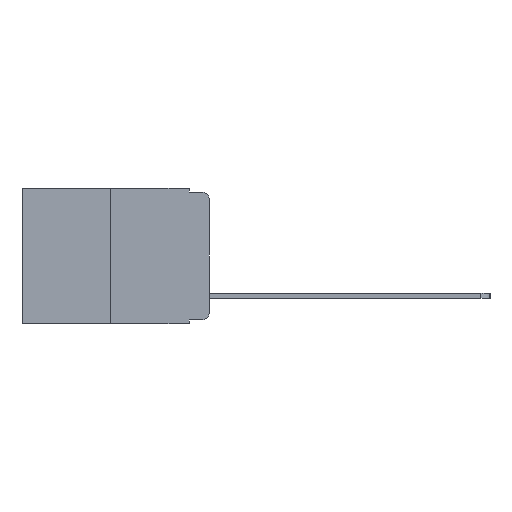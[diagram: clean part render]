
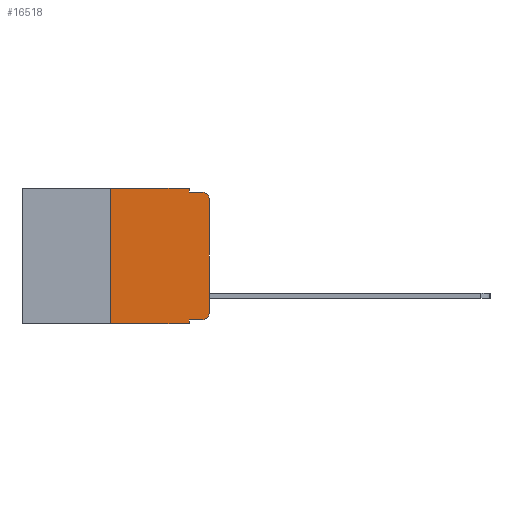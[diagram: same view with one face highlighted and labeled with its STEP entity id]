
A CAD part, left-side view. The second image highlights one B-rep face of the part: STEP entity #16518.
In plain terms, the highlighted planar face has unit normal (-1, 0, 0).
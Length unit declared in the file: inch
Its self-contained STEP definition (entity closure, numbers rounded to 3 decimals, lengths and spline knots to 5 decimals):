
#79 = ORIENTED_EDGE ( 'NONE', *, *, #9036, .T. ) ;
#179 = VERTEX_POINT ( 'NONE', #13125 ) ;
#211 = ORIENTED_EDGE ( 'NONE', *, *, #16950, .T. ) ;
#239 = CARTESIAN_POINT ( 'NONE',  ( 0., 0.051, -0.333 ) ) ;
#709 = ORIENTED_EDGE ( 'NONE', *, *, #10449, .F. ) ;
#715 = EDGE_CURVE ( 'NONE', #5940, #3988, #12604, .T. ) ;
#800 = LINE ( 'NONE', #12692, #12068 ) ;
#930 = ORIENTED_EDGE ( 'NONE', *, *, #10160, .T. ) ;
#963 = ORIENTED_EDGE ( 'NONE', *, *, #4526, .F. ) ;
#1003 = CARTESIAN_POINT ( 'NONE',  ( 0., 0.25, -0.343 ) ) ;
#1034 = ORIENTED_EDGE ( 'NONE', *, *, #6282, .F. ) ;
#1177 = VERTEX_POINT ( 'NONE', #4292 ) ;
#1262 = ORIENTED_EDGE ( 'NONE', *, *, #2273, .F. ) ;
#1403 = ORIENTED_EDGE ( 'NONE', *, *, #5444, .F. ) ;
#1553 = ORIENTED_EDGE ( 'NONE', *, *, #715, .T. ) ;
#1804 = VERTEX_POINT ( 'NONE', #2269 ) ;
#1858 = PLANE ( 'NONE',  #3168 ) ;
#1909 = ORIENTED_EDGE ( 'NONE', *, *, #4482, .T. ) ;
#2108 = VECTOR ( 'NONE', #14297, 39.37008 ) ;
#2269 = CARTESIAN_POINT ( 'NONE',  ( 0., 0.051, 0. ) ) ;
#2273 = EDGE_CURVE ( 'NONE', #1804, #179, #9886, .T. ) ;
#2800 = DIRECTION ( 'NONE',  ( -1., 0., 0. ) ) ;
#3168 = AXIS2_PLACEMENT_3D ( 'NONE', #4656, #11345, #3285 ) ;
#3285 = DIRECTION ( 'NONE',  ( 0., 0., -1. ) ) ;
#3413 = CARTESIAN_POINT ( 'NONE',  ( 0., 0.02, -0.03 ) ) ;
#3469 = LINE ( 'NONE', #12544, #3921 ) ;
#3643 = AXIS2_PLACEMENT_3D ( 'NONE', #3413, #3991, #3996 ) ;
#3776 = VERTEX_POINT ( 'NONE', #10372 ) ;
#3800 = DIRECTION ( 'NONE',  ( 0., 0., -1. ) ) ;
#3864 = LINE ( 'NONE', #9375, #10582 ) ;
#3921 = VECTOR ( 'NONE', #4580, 39.37008 ) ;
#3988 = VERTEX_POINT ( 'NONE', #6637 ) ;
#3991 = DIRECTION ( 'NONE',  ( -1., 0., 0. ) ) ;
#3996 = DIRECTION ( 'NONE',  ( 0., 0., -1. ) ) ;
#4260 = CARTESIAN_POINT ( 'NONE',  ( 0., 0., -0.03 ) ) ;
#4292 = CARTESIAN_POINT ( 'NONE',  ( 0., 0., -0.313 ) ) ;
#4482 = EDGE_CURVE ( 'NONE', #1177, #5940, #6712, .T. ) ;
#4526 = EDGE_CURVE ( 'NONE', #9452, #5182, #9406, .T. ) ;
#4580 = DIRECTION ( 'NONE',  ( 0., -1., 0. ) ) ;
#4656 = CARTESIAN_POINT ( 'NONE',  ( 0., 0.473, 0. ) ) ;
#5182 = VERTEX_POINT ( 'NONE', #15541 ) ;
#5329 = EDGE_LOOP ( 'NONE', ( #1909, #1553, #1403, #1262, #1034, #963, #930, #709, #211, #79 ) ) ;
#5444 = EDGE_CURVE ( 'NONE', #179, #3988, #9373, .T. ) ;
#5659 = VECTOR ( 'NONE', #9427, 39.37008 ) ;
#5940 = VERTEX_POINT ( 'NONE', #4260 ) ;
#6282 = EDGE_CURVE ( 'NONE', #5182, #1804, #3864, .T. ) ;
#6637 = CARTESIAN_POINT ( 'NONE',  ( 0., 0.02, -0.01 ) ) ;
#6712 = LINE ( 'NONE', #17140, #16820 ) ;
#7414 = DIRECTION ( 'NONE',  ( 0., 0., -1. ) ) ;
#8039 = CIRCLE ( 'NONE', #10532, 0.02 ) ;
#8192 = CARTESIAN_POINT ( 'NONE',  ( 0., 0.473, -0.343 ) ) ;
#9036 = EDGE_CURVE ( 'NONE', #13520, #1177, #8039, .T. ) ;
#9291 = DIRECTION ( 'NONE',  ( 0., 0., 1. ) ) ;
#9373 = LINE ( 'NONE', #15152, #2108 ) ;
#9375 = CARTESIAN_POINT ( 'NONE',  ( 0., 0.473, 0. ) ) ;
#9406 = LINE ( 'NONE', #11432, #9811 ) ;
#9427 = DIRECTION ( 'NONE',  ( 0., -1., 0. ) ) ;
#9452 = VERTEX_POINT ( 'NONE', #1003 ) ;
#9489 = VECTOR ( 'NONE', #3800, 39.37008 ) ;
#9636 = DIRECTION ( 'NONE',  ( 0., -1., 0. ) ) ;
#9811 = VECTOR ( 'NONE', #11868, 39.37008 ) ;
#9886 = LINE ( 'NONE', #12912, #9489 ) ;
#10160 = EDGE_CURVE ( 'NONE', #9452, #3776, #16623, .T. ) ;
#10372 = CARTESIAN_POINT ( 'NONE',  ( 0., 0.051, -0.343 ) ) ;
#10449 = EDGE_CURVE ( 'NONE', #11230, #3776, #800, .T. ) ;
#10532 = AXIS2_PLACEMENT_3D ( 'NONE', #10914, #2800, #12222 ) ;
#10582 = VECTOR ( 'NONE', #9636, 39.37008 ) ;
#10914 = CARTESIAN_POINT ( 'NONE',  ( 0., 0.02, -0.313 ) ) ;
#11230 = VERTEX_POINT ( 'NONE', #239 ) ;
#11345 = DIRECTION ( 'NONE',  ( 1., 0., 0. ) ) ;
#11432 = CARTESIAN_POINT ( 'NONE',  ( 0., 0.25, 0. ) ) ;
#11868 = DIRECTION ( 'NONE',  ( 0., 0., 1. ) ) ;
#12068 = VECTOR ( 'NONE', #7414, 39.37008 ) ;
#12222 = DIRECTION ( 'NONE',  ( 0., 0., -1. ) ) ;
#12544 = CARTESIAN_POINT ( 'NONE',  ( 0., 0.051, -0.333 ) ) ;
#12604 = CIRCLE ( 'NONE', #3643, 0.02 ) ;
#12692 = CARTESIAN_POINT ( 'NONE',  ( 0., 0.051, 0. ) ) ;
#12912 = CARTESIAN_POINT ( 'NONE',  ( 0., 0.051, 0. ) ) ;
#13125 = CARTESIAN_POINT ( 'NONE',  ( 0., 0.051, -0.01 ) ) ;
#13520 = VERTEX_POINT ( 'NONE', #16624 ) ;
#14151 = FACE_OUTER_BOUND ( 'NONE', #5329, .T. ) ;
#14297 = DIRECTION ( 'NONE',  ( 0., -1., 0. ) ) ;
#15152 = CARTESIAN_POINT ( 'NONE',  ( 0., 0.051, -0.01 ) ) ;
#15541 = CARTESIAN_POINT ( 'NONE',  ( 0., 0.25, 0. ) ) ;
#16518 = ADVANCED_FACE ( 'NONE', ( #14151 ), #1858, .F. ) ;
#16623 = LINE ( 'NONE', #8192, #5659 ) ;
#16624 = CARTESIAN_POINT ( 'NONE',  ( 0., 0.02, -0.333 ) ) ;
#16820 = VECTOR ( 'NONE', #9291, 39.37008 ) ;
#16950 = EDGE_CURVE ( 'NONE', #11230, #13520, #3469, .T. ) ;
#17140 = CARTESIAN_POINT ( 'NONE',  ( 0., 0., 0. ) ) ;
